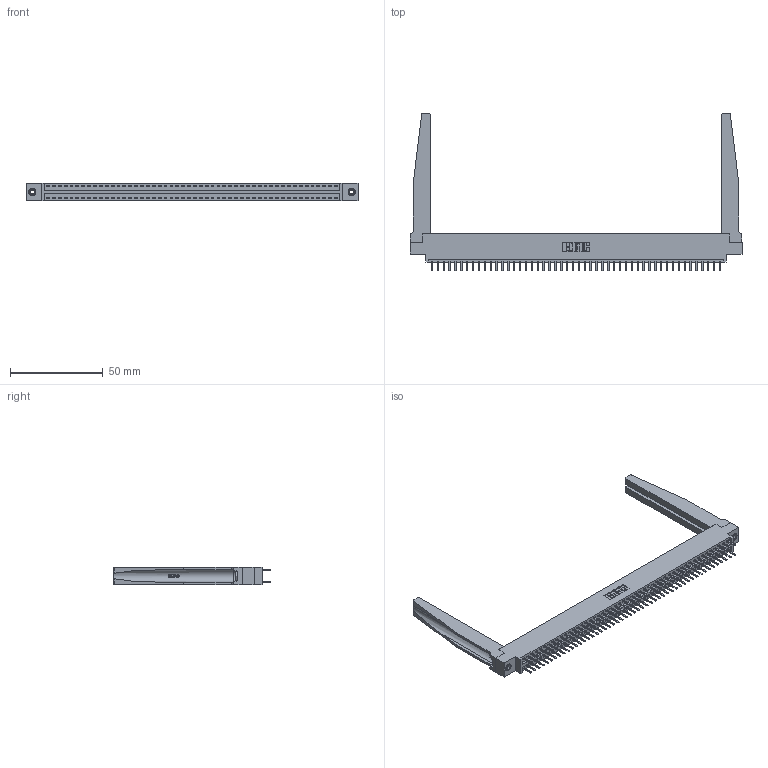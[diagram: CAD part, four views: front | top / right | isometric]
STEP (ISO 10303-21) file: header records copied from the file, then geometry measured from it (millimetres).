
FILE_DESCRIPTION (( 'STEP AP203' ), '1' );
FILE_NAME ('396-100-520-878.STEP', '2019-11-02T17:21:39', ( '' ), ( '' ), 'SwSTEP 2.0', 'SolidWorks 2016', '' );
FILE_SCHEMA (( 'CONFIG_CONTROL_DESIGN' ));
Length unit declared in the file: inch
Products named in the file (5): 346-220-078_345-220-078; 345-250-001_345-250-001-102; 396-100-520-878; 346 Part_0.170 Offset - 0.156 Dia-TH; 345-292-001_345-293-120
Assembly tree (105 placements, depth 2):
  396-100-520-878
    346 Part_0.170 Offset - 0.156 Dia-TH
    345-292-001_345-293-120  x100
    346-220-078_345-220-078  x2
    345-250-001_345-250-001-102  x2
Bounding box: 179.32 x 85.29 x 9.4 mm (x, y, z)
Volume: 24258.7 mm3; surface area: 30588.4 mm2
Topology: 105 solids, 105 shells, 5960 faces, 17249 edges, 11222 vertices
Faces by surface type: plane 3922, cylinder 1986, bspline 36, cone 12, torus 4
Entity records: 36548 total; most frequent: CARTESIAN_POINT 6963, ORIENTED_EDGE 5774, DIRECTION 5161, EDGE_CURVE 2887, VECTOR 2457, LINE 2457, VERTEX_POINT 1916, AXIS2_PLACEMENT_3D 1352
